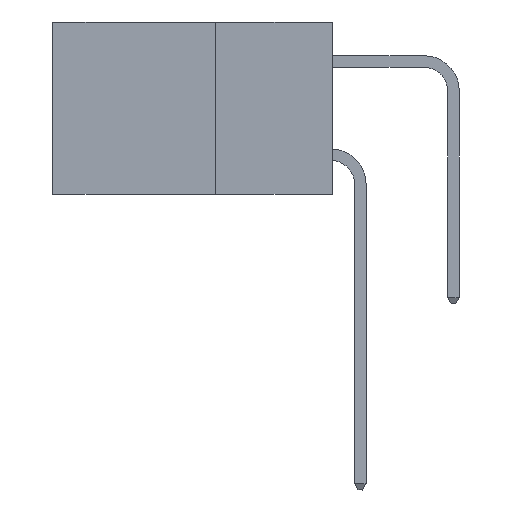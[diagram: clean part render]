
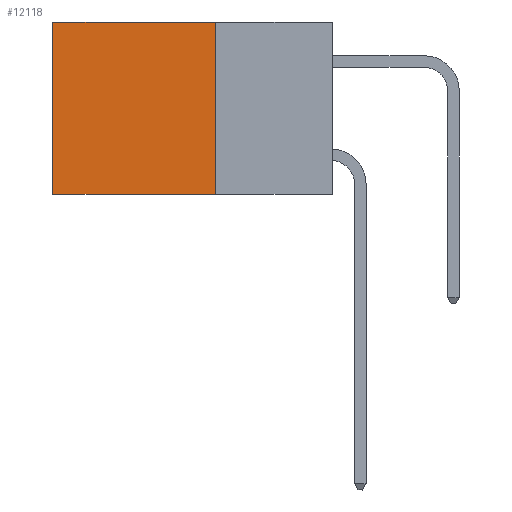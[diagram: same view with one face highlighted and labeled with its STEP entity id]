
A CAD part, left-side view. The second image highlights one B-rep face of the part: STEP entity #12118.
In plain terms, the highlighted planar face has unit normal (-1, 0, 0).
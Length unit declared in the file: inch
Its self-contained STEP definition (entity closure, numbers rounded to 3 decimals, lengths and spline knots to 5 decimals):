
#234 = DIRECTION ( 'NONE',  ( 0., 0., -1. ) ) ;
#332 = VECTOR ( 'NONE', #4598, 39.37008 ) ;
#378 = EDGE_LOOP ( 'NONE', ( #2541, #12180, #20175, #13861 ) ) ;
#738 = DIRECTION ( 'NONE',  ( 0., 1., 0. ) ) ;
#1362 = PLANE ( 'NONE',  #8055 ) ;
#1521 = CARTESIAN_POINT ( 'NONE',  ( 0.2615, 0.25, 0. ) ) ;
#2011 = LINE ( 'NONE', #19641, #2342 ) ;
#2342 = VECTOR ( 'NONE', #234, 39.37008 ) ;
#2541 = ORIENTED_EDGE ( 'NONE', *, *, #10468, .T. ) ;
#2767 = CARTESIAN_POINT ( 'NONE',  ( 0.2615, 0.6, -0.37 ) ) ;
#2864 = LINE ( 'NONE', #22385, #6650 ) ;
#3146 = FACE_OUTER_BOUND ( 'NONE', #378, .T. ) ;
#3764 = CARTESIAN_POINT ( 'NONE',  ( 0.2615, 0.6, -0.37 ) ) ;
#4598 = DIRECTION ( 'NONE',  ( 0., 1., 0. ) ) ;
#4937 = EDGE_CURVE ( 'NONE', #14834, #7193, #11917, .T. ) ;
#6408 = VERTEX_POINT ( 'NONE', #1521 ) ;
#6650 = VECTOR ( 'NONE', #738, 39.37008 ) ;
#7193 = VERTEX_POINT ( 'NONE', #2767 ) ;
#7244 = VECTOR ( 'NONE', #18170, 39.37008 ) ;
#7904 = EDGE_CURVE ( 'NONE', #6408, #14834, #2011, .T. ) ;
#8055 = AXIS2_PLACEMENT_3D ( 'NONE', #12231, #8673, #8550 ) ;
#8117 = CARTESIAN_POINT ( 'NONE',  ( 0.2615, 0.25, -0.37 ) ) ;
#8550 = DIRECTION ( 'NONE',  ( 0., 0., -1. ) ) ;
#8673 = DIRECTION ( 'NONE',  ( 1., 0., 0. ) ) ;
#10468 = EDGE_CURVE ( 'NONE', #17897, #7193, #21846, .T. ) ;
#11917 = LINE ( 'NONE', #20792, #332 ) ;
#12118 = ADVANCED_FACE ( 'NONE', ( #3146 ), #1362, .F. ) ;
#12180 = ORIENTED_EDGE ( 'NONE', *, *, #4937, .F. ) ;
#12231 = CARTESIAN_POINT ( 'NONE',  ( 0.2615, 0.25, -0.37 ) ) ;
#13861 = ORIENTED_EDGE ( 'NONE', *, *, #21428, .T. ) ;
#14624 = CARTESIAN_POINT ( 'NONE',  ( 0.2615, 0.6, 0. ) ) ;
#14834 = VERTEX_POINT ( 'NONE', #8117 ) ;
#17897 = VERTEX_POINT ( 'NONE', #14624 ) ;
#18170 = DIRECTION ( 'NONE',  ( 0., 0., -1. ) ) ;
#19641 = CARTESIAN_POINT ( 'NONE',  ( 0.2615, 0.25, -0.37 ) ) ;
#20175 = ORIENTED_EDGE ( 'NONE', *, *, #7904, .F. ) ;
#20792 = CARTESIAN_POINT ( 'NONE',  ( 0.2615, 0.25, -0.37 ) ) ;
#21428 = EDGE_CURVE ( 'NONE', #6408, #17897, #2864, .T. ) ;
#21846 = LINE ( 'NONE', #3764, #7244 ) ;
#22385 = CARTESIAN_POINT ( 'NONE',  ( 0.2615, 0.25, 0. ) ) ;
